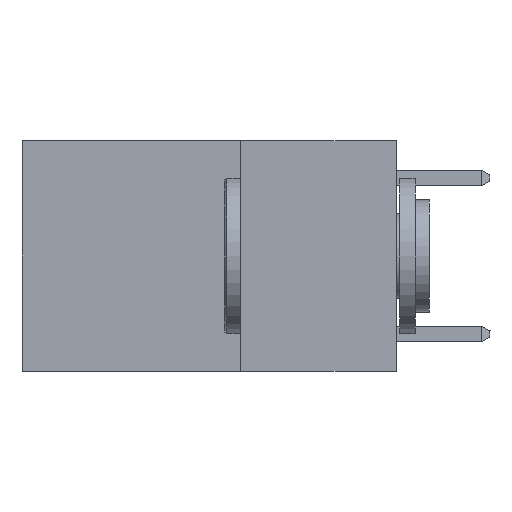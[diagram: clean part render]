
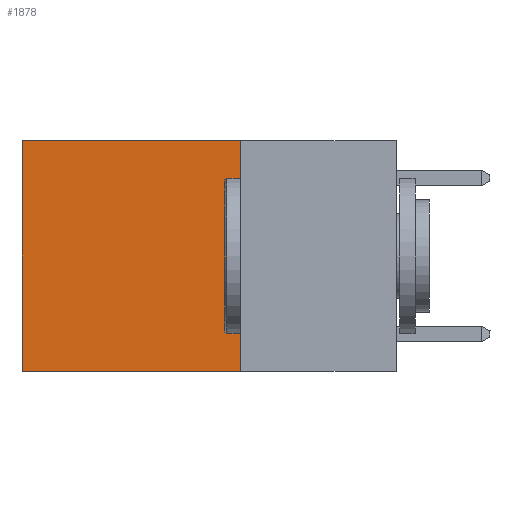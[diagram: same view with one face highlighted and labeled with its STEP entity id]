
A CAD part, left-side view. The second image highlights one B-rep face of the part: STEP entity #1878.
In plain terms, the highlighted planar face has unit normal (-1, 0, 0).
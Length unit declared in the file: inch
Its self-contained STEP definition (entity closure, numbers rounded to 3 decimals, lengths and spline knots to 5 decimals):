
#1464 = EDGE_CURVE ( 'NONE', #7579, #13726, #20882, .T. ) ;
#1653 = DIRECTION ( 'NONE',  ( 0., 1., 0. ) ) ;
#1878 = ADVANCED_FACE ( 'NONE', ( #16284 ), #2973, .F. ) ;
#2973 = PLANE ( 'NONE',  #9049 ) ;
#3072 = VECTOR ( 'NONE', #26878, 39.37008 ) ;
#3818 = LINE ( 'NONE', #29203, #3072 ) ;
#3831 = ORIENTED_EDGE ( 'NONE', *, *, #1464, .T. ) ;
#4930 = LINE ( 'NONE', #26564, #29820 ) ;
#5016 = ORIENTED_EDGE ( 'NONE', *, *, #6896, .F. ) ;
#5051 = VERTEX_POINT ( 'NONE', #9539 ) ;
#5345 = DIRECTION ( 'NONE',  ( 1., 0., 0. ) ) ;
#6896 = EDGE_CURVE ( 'NONE', #5051, #27323, #8642, .T. ) ;
#7579 = VERTEX_POINT ( 'NONE', #14469 ) ;
#8245 = ORIENTED_EDGE ( 'NONE', *, *, #11465, .F. ) ;
#8380 = VECTOR ( 'NONE', #1653, 39.37008 ) ;
#8642 = LINE ( 'NONE', #18067, #8380 ) ;
#9049 = AXIS2_PLACEMENT_3D ( 'NONE', #12395, #5345, #21770 ) ;
#9539 = CARTESIAN_POINT ( 'NONE',  ( 0.2625, 0.25, -0.37 ) ) ;
#10602 = ORIENTED_EDGE ( 'NONE', *, *, #25235, .T. ) ;
#11465 = EDGE_CURVE ( 'NONE', #7579, #5051, #3818, .T. ) ;
#12395 = CARTESIAN_POINT ( 'NONE',  ( 0.2625, 0.25, 0. ) ) ;
#13726 = VERTEX_POINT ( 'NONE', #25805 ) ;
#14469 = CARTESIAN_POINT ( 'NONE',  ( 0.2625, 0.25, 0. ) ) ;
#16284 = FACE_OUTER_BOUND ( 'NONE', #21824, .T. ) ;
#18067 = CARTESIAN_POINT ( 'NONE',  ( 0.2625, 0.25, -0.37 ) ) ;
#19567 = CARTESIAN_POINT ( 'NONE',  ( 0.2625, 0.6, -0.37 ) ) ;
#20510 = VECTOR ( 'NONE', #29740, 39.37008 ) ;
#20882 = LINE ( 'NONE', #22756, #20510 ) ;
#21770 = DIRECTION ( 'NONE',  ( 0., 0., -1. ) ) ;
#21824 = EDGE_LOOP ( 'NONE', ( #10602, #5016, #8245, #3831 ) ) ;
#22756 = CARTESIAN_POINT ( 'NONE',  ( 0.2625, 0.25, 0. ) ) ;
#25235 = EDGE_CURVE ( 'NONE', #13726, #27323, #4930, .T. ) ;
#25805 = CARTESIAN_POINT ( 'NONE',  ( 0.2625, 0.6, 0. ) ) ;
#26564 = CARTESIAN_POINT ( 'NONE',  ( 0.2625, 0.6, 0. ) ) ;
#26878 = DIRECTION ( 'NONE',  ( 0., 0., -1. ) ) ;
#27323 = VERTEX_POINT ( 'NONE', #19567 ) ;
#28919 = DIRECTION ( 'NONE',  ( 0., 0., -1. ) ) ;
#29203 = CARTESIAN_POINT ( 'NONE',  ( 0.2625, 0.25, 0. ) ) ;
#29740 = DIRECTION ( 'NONE',  ( 0., 1., 0. ) ) ;
#29820 = VECTOR ( 'NONE', #28919, 39.37008 ) ;
